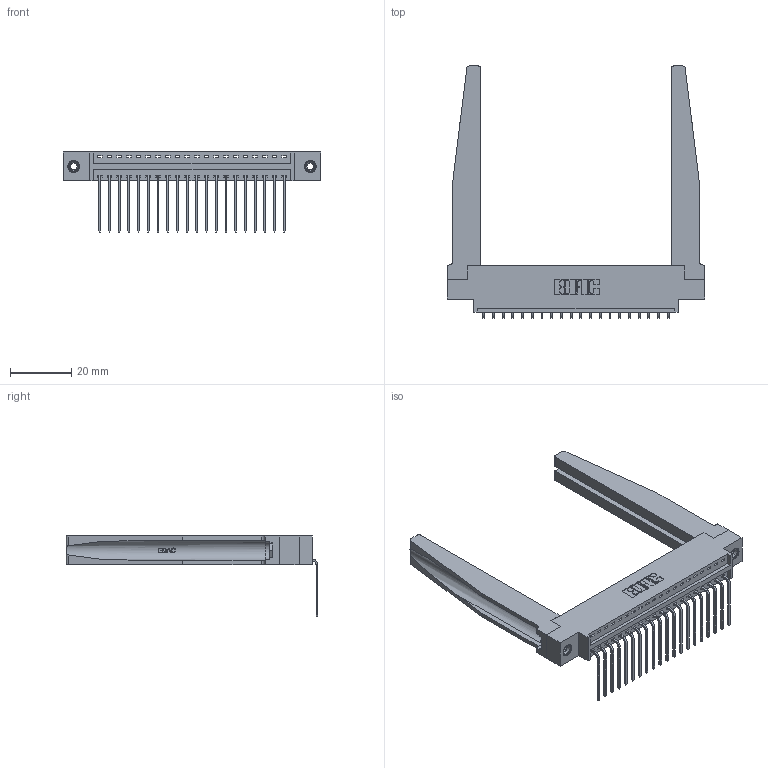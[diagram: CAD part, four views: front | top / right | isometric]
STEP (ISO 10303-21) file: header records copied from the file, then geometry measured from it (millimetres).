
FILE_DESCRIPTION (( 'STEP AP203' ), '1' );
FILE_NAME ('396-020-559-678.STEP', '2019-10-31T21:00:18', ( '' ), ( '' ), 'SwSTEP 2.0', 'SolidWorks 2016', '' );
FILE_SCHEMA (( 'CONFIG_CONTROL_DESIGN' ));
Length unit declared in the file: inch
Products named in the file (5): 346 Part_0.170 Offset - 0.156 Dia-TH; 345-292-001_558 559 Tail - 1; 346-220-078_345-220-078; 345-250-001_345-250-001-102; 396-020-559-678
Assembly tree (25 placements, depth 2):
  396-020-559-678
    346 Part_0.170 Offset - 0.156 Dia-TH
    345-292-001_558 559 Tail - 1  x20
    346-220-078_345-220-078  x2
    345-250-001_345-250-001-102  x2
Bounding box: 84.07 x 82.36 x 26.16 mm (x, y, z)
Volume: 14717 mm3; surface area: 16619.8 mm2
Topology: 25 solids, 25 shells, 1560 faces, 4589 edges, 3022 vertices
Faces by surface type: plane 1062, cylinder 446, bspline 36, cone 12, torus 4
Entity records: 20338 total; most frequent: CARTESIAN_POINT 4407, ORIENTED_EDGE 3250, DIRECTION 2899, EDGE_CURVE 1625, VECTOR 1319, LINE 1319, VERTEX_POINT 1076, AXIS2_PLACEMENT_3D 790
